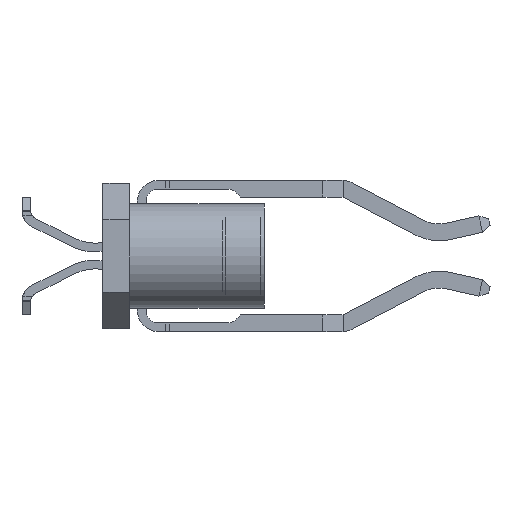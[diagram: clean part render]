
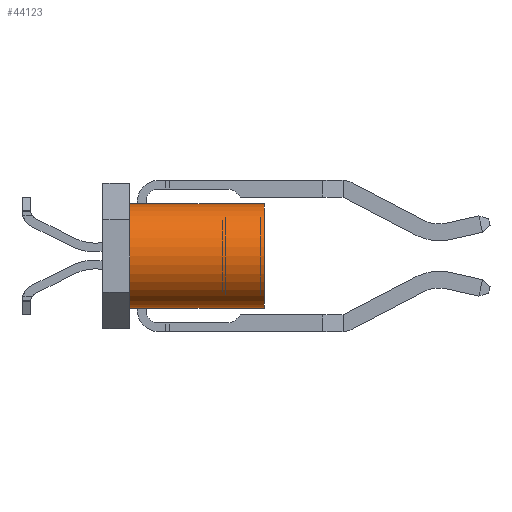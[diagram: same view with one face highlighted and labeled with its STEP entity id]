
A CAD part, left-side view. The second image highlights one B-rep face of the part: STEP entity #44123.
In plain terms, the highlighted cylindrical face has radius 1.968 mm (diameter 3.937 mm), a partial arc.
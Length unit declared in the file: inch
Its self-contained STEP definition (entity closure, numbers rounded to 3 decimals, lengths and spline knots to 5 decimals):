
#846 = ORIENTED_EDGE ( 'NONE', *, *, #46889, .F. ) ;
#1720 = ORIENTED_EDGE ( 'NONE', *, *, #7958, .T. ) ;
#3515 = ORIENTED_EDGE ( 'NONE', *, *, #32074, .F. ) ;
#4816 = VERTEX_POINT ( 'NONE', #17446 ) ;
#6448 = CIRCLE ( 'NONE', #9459, 0.0775 ) ;
#7958 = EDGE_CURVE ( 'NONE', #41143, #42027, #37745, .T. ) ;
#9020 = DIRECTION ( 'NONE',  ( 0., -1., 0. ) ) ;
#9459 = AXIS2_PLACEMENT_3D ( 'NONE', #28463, #24770, #31680 ) ;
#11414 = CARTESIAN_POINT ( 'NONE',  ( 0., 0.04, -0.0775 ) ) ;
#15790 = DIRECTION ( 'NONE',  ( 0., 1., 0. ) ) ;
#17404 = VERTEX_POINT ( 'NONE', #19598 ) ;
#17446 = CARTESIAN_POINT ( 'NONE',  ( 0., 0.24, 0.0775 ) ) ;
#18584 = CARTESIAN_POINT ( 'NONE',  ( 0., 0.24, 0. ) ) ;
#19472 = CARTESIAN_POINT ( 'NONE',  ( 0., 0.24, -0.0775 ) ) ;
#19598 = CARTESIAN_POINT ( 'NONE',  ( 0., 0.24, -0.0775 ) ) ;
#20761 = ORIENTED_EDGE ( 'NONE', *, *, #28348, .T. ) ;
#20922 = LINE ( 'NONE', #21258, #31247 ) ;
#21258 = CARTESIAN_POINT ( 'NONE',  ( 0., 0.24, 0.0775 ) ) ;
#22281 = DIRECTION ( 'NONE',  ( 0., -1., 0. ) ) ;
#24770 = DIRECTION ( 'NONE',  ( 0., 1., 0. ) ) ;
#26949 = CYLINDRICAL_SURFACE ( 'NONE', #33740, 0.0775 ) ;
#28348 = EDGE_CURVE ( 'NONE', #17404, #41143, #31545, .T. ) ;
#28463 = CARTESIAN_POINT ( 'NONE',  ( 0., 0.24, 0. ) ) ;
#28699 = VECTOR ( 'NONE', #9020, 39.37008 ) ;
#31247 = VECTOR ( 'NONE', #32315, 39.37008 ) ;
#31545 = LINE ( 'NONE', #19472, #28699 ) ;
#31680 = DIRECTION ( 'NONE',  ( 0., 0., 1. ) ) ;
#32074 = EDGE_CURVE ( 'NONE', #17404, #4816, #6448, .T. ) ;
#32315 = DIRECTION ( 'NONE',  ( 0., -1., 0. ) ) ;
#33740 = AXIS2_PLACEMENT_3D ( 'NONE', #18584, #22281, #37176 ) ;
#35963 = CARTESIAN_POINT ( 'NONE',  ( 0., 0.04, 0.0775 ) ) ;
#37176 = DIRECTION ( 'NONE',  ( 0., 0., -1. ) ) ;
#37745 = CIRCLE ( 'NONE', #45619, 0.0775 ) ;
#39533 = FACE_OUTER_BOUND ( 'NONE', #47460, .T. ) ;
#41131 = DIRECTION ( 'NONE',  ( 0., 0., 1. ) ) ;
#41143 = VERTEX_POINT ( 'NONE', #11414 ) ;
#42027 = VERTEX_POINT ( 'NONE', #35963 ) ;
#44123 = ADVANCED_FACE ( 'NONE', ( #39533 ), #26949, .T. ) ;
#44829 = CARTESIAN_POINT ( 'NONE',  ( 0., 0.04, 0. ) ) ;
#45619 = AXIS2_PLACEMENT_3D ( 'NONE', #44829, #15790, #41131 ) ;
#46889 = EDGE_CURVE ( 'NONE', #4816, #42027, #20922, .T. ) ;
#47460 = EDGE_LOOP ( 'NONE', ( #846, #3515, #20761, #1720 ) ) ;
